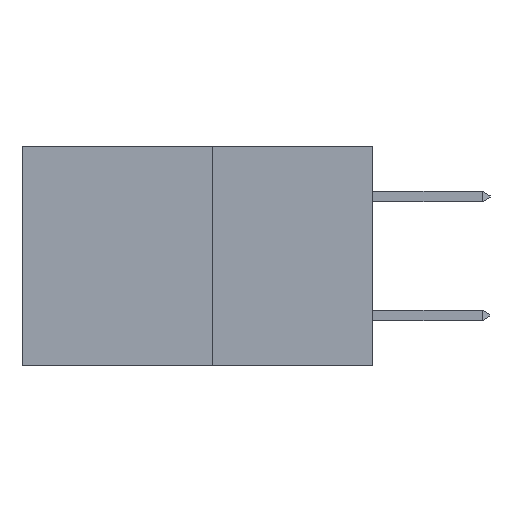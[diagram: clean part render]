
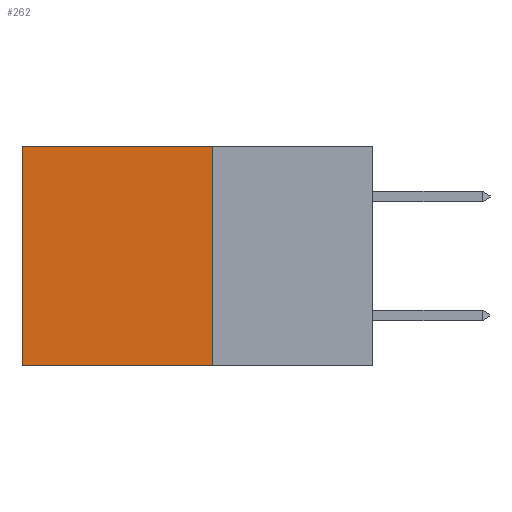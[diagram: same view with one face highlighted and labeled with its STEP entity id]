
A CAD part, left-side view. The second image highlights one B-rep face of the part: STEP entity #262.
In plain terms, the highlighted planar face has unit normal (-1, 0, 0).
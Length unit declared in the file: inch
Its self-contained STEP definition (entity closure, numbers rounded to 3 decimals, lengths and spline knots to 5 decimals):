
#245 = LINE ( 'NONE', #5649, #5980 ) ;
#262 = ADVANCED_FACE ( 'NONE', ( #3095 ), #9503, .F. ) ;
#358 = EDGE_CURVE ( 'NONE', #5241, #3706, #4457, .T. ) ;
#1684 = AXIS2_PLACEMENT_3D ( 'NONE', #7628, #9482, #2564 ) ;
#2281 = EDGE_CURVE ( 'NONE', #5453, #5068, #245, .T. ) ;
#2564 = DIRECTION ( 'NONE',  ( 0., 0., -1. ) ) ;
#2700 = ORIENTED_EDGE ( 'NONE', *, *, #2281, .T. ) ;
#3021 = CARTESIAN_POINT ( 'NONE',  ( 0.277, 0.27, -0.37 ) ) ;
#3060 = EDGE_CURVE ( 'NONE', #5453, #5241, #9133, .T. ) ;
#3095 = FACE_OUTER_BOUND ( 'NONE', #4484, .T. ) ;
#3693 = CARTESIAN_POINT ( 'NONE',  ( 0.277, 0.27, -0.37 ) ) ;
#3706 = VERTEX_POINT ( 'NONE', #4862 ) ;
#4042 = DIRECTION ( 'NONE',  ( 0., 1., 0. ) ) ;
#4457 = LINE ( 'NONE', #7414, #8081 ) ;
#4484 = EDGE_LOOP ( 'NONE', ( #4540, #7264, #9425, #2700 ) ) ;
#4540 = ORIENTED_EDGE ( 'NONE', *, *, #6113, .T. ) ;
#4862 = CARTESIAN_POINT ( 'NONE',  ( 0.277, 0.59, -0.37 ) ) ;
#5068 = VERTEX_POINT ( 'NONE', #5512 ) ;
#5241 = VERTEX_POINT ( 'NONE', #3021 ) ;
#5453 = VERTEX_POINT ( 'NONE', #5872 ) ;
#5512 = CARTESIAN_POINT ( 'NONE',  ( 0.277, 0.59, 0. ) ) ;
#5629 = VECTOR ( 'NONE', #9282, 39.37008 ) ;
#5649 = CARTESIAN_POINT ( 'NONE',  ( 0.277, 0.27, 0. ) ) ;
#5872 = CARTESIAN_POINT ( 'NONE',  ( 0.277, 0.27, 0. ) ) ;
#5980 = VECTOR ( 'NONE', #4042, 39.37008 ) ;
#6113 = EDGE_CURVE ( 'NONE', #5068, #3706, #9186, .T. ) ;
#6685 = DIRECTION ( 'NONE',  ( 0., 1., 0. ) ) ;
#7264 = ORIENTED_EDGE ( 'NONE', *, *, #358, .F. ) ;
#7357 = VECTOR ( 'NONE', #8250, 39.37008 ) ;
#7414 = CARTESIAN_POINT ( 'NONE',  ( 0.277, 0.27, -0.37 ) ) ;
#7628 = CARTESIAN_POINT ( 'NONE',  ( 0.277, 0.27, -0.37 ) ) ;
#8081 = VECTOR ( 'NONE', #6685, 39.37008 ) ;
#8243 = CARTESIAN_POINT ( 'NONE',  ( 0.277, 0.59, -0.37 ) ) ;
#8250 = DIRECTION ( 'NONE',  ( 0., 0., -1. ) ) ;
#9133 = LINE ( 'NONE', #3693, #5629 ) ;
#9186 = LINE ( 'NONE', #8243, #7357 ) ;
#9282 = DIRECTION ( 'NONE',  ( 0., 0., -1. ) ) ;
#9425 = ORIENTED_EDGE ( 'NONE', *, *, #3060, .F. ) ;
#9482 = DIRECTION ( 'NONE',  ( 1., 0., 0. ) ) ;
#9503 = PLANE ( 'NONE',  #1684 ) ;
